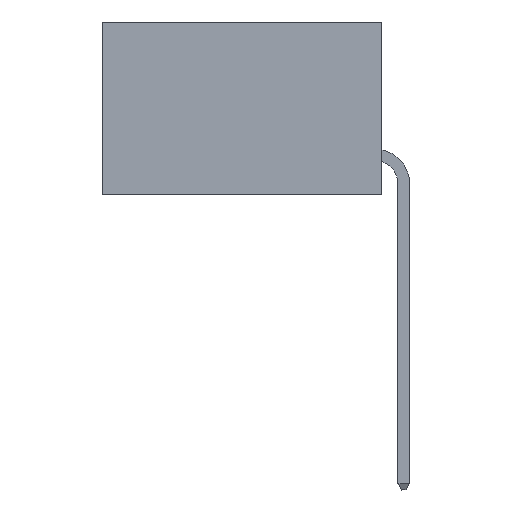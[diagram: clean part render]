
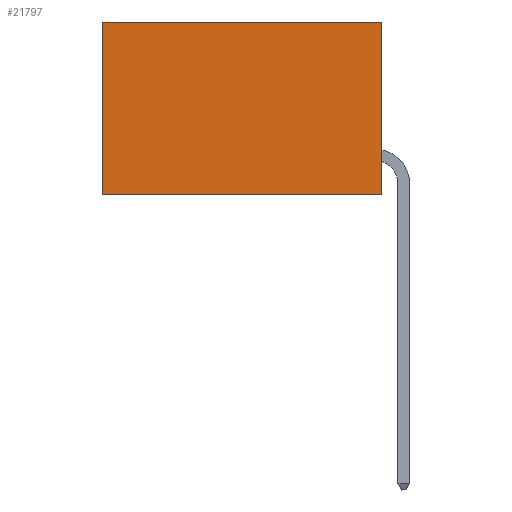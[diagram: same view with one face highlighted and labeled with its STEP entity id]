
A CAD part, left-side view. The second image highlights one B-rep face of the part: STEP entity #21797.
In plain terms, the highlighted planar face has unit normal (-1, 0, 0).
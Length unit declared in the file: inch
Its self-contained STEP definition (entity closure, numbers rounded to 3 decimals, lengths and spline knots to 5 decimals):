
#1270 = CARTESIAN_POINT ( 'NONE',  ( 0.2875, 0., 0. ) ) ;
#1480 = VECTOR ( 'NONE', #22150, 39.37008 ) ;
#1802 = ORIENTED_EDGE ( 'NONE', *, *, #3109, .T. ) ;
#1890 = DIRECTION ( 'NONE',  ( 0., 1., 0. ) ) ;
#2028 = LINE ( 'NONE', #3470, #1480 ) ;
#3109 = EDGE_CURVE ( 'NONE', #43623, #42180, #5285, .T. ) ;
#3470 = CARTESIAN_POINT ( 'NONE',  ( 0.2875, 0., 0. ) ) ;
#3982 = ORIENTED_EDGE ( 'NONE', *, *, #41857, .F. ) ;
#4802 = DIRECTION ( 'NONE',  ( 0., 0., -1. ) ) ;
#5268 = EDGE_LOOP ( 'NONE', ( #1802, #42205, #3982, #40891 ) ) ;
#5285 = LINE ( 'NONE', #30644, #7494 ) ;
#5901 = AXIS2_PLACEMENT_3D ( 'NONE', #44070, #26277, #4802 ) ;
#7494 = VECTOR ( 'NONE', #20346, 39.37008 ) ;
#7878 = VECTOR ( 'NONE', #33548, 39.37008 ) ;
#12639 = CARTESIAN_POINT ( 'NONE',  ( 0.2875, 0., -0.37 ) ) ;
#13194 = CARTESIAN_POINT ( 'NONE',  ( 0.2875, 0., 0. ) ) ;
#13312 = CARTESIAN_POINT ( 'NONE',  ( 0.2875, 0., -0.37 ) ) ;
#17562 = CARTESIAN_POINT ( 'NONE',  ( 0.2875, 0.6, -0.37 ) ) ;
#20346 = DIRECTION ( 'NONE',  ( 0., 0., -1. ) ) ;
#21797 = ADVANCED_FACE ( 'NONE', ( #37359 ), #30035, .F. ) ;
#22150 = DIRECTION ( 'NONE',  ( 0., 0., -1. ) ) ;
#26277 = DIRECTION ( 'NONE',  ( 1., 0., 0. ) ) ;
#26332 = LINE ( 'NONE', #1270, #7878 ) ;
#30035 = PLANE ( 'NONE',  #5901 ) ;
#30644 = CARTESIAN_POINT ( 'NONE',  ( 0.2875, 0.6, 0. ) ) ;
#30803 = LINE ( 'NONE', #12639, #39180 ) ;
#31835 = CARTESIAN_POINT ( 'NONE',  ( 0.2875, 0.6, 0. ) ) ;
#33548 = DIRECTION ( 'NONE',  ( 0., 1., 0. ) ) ;
#34135 = EDGE_CURVE ( 'NONE', #36482, #43623, #26332, .T. ) ;
#35822 = EDGE_CURVE ( 'NONE', #44018, #42180, #30803, .T. ) ;
#36482 = VERTEX_POINT ( 'NONE', #13194 ) ;
#37359 = FACE_OUTER_BOUND ( 'NONE', #5268, .T. ) ;
#39180 = VECTOR ( 'NONE', #1890, 39.37008 ) ;
#40891 = ORIENTED_EDGE ( 'NONE', *, *, #34135, .T. ) ;
#41857 = EDGE_CURVE ( 'NONE', #36482, #44018, #2028, .T. ) ;
#42180 = VERTEX_POINT ( 'NONE', #17562 ) ;
#42205 = ORIENTED_EDGE ( 'NONE', *, *, #35822, .F. ) ;
#43623 = VERTEX_POINT ( 'NONE', #31835 ) ;
#44018 = VERTEX_POINT ( 'NONE', #13312 ) ;
#44070 = CARTESIAN_POINT ( 'NONE',  ( 0.2875, 0., 0. ) ) ;
